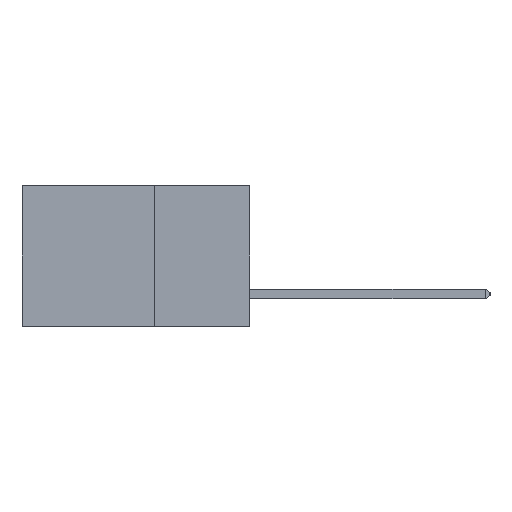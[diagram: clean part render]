
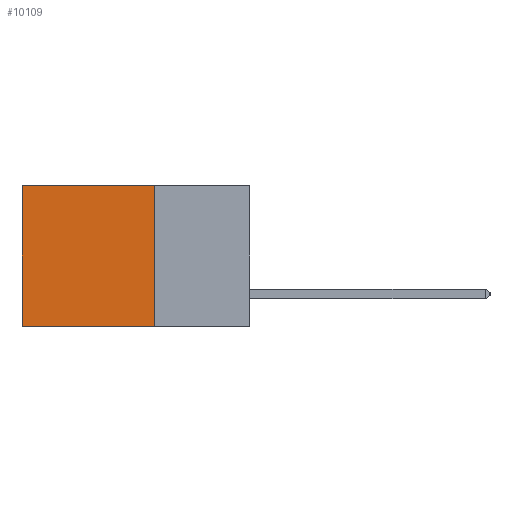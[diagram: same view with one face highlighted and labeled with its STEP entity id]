
A CAD part, left-side view. The second image highlights one B-rep face of the part: STEP entity #10109.
In plain terms, the highlighted planar face has unit normal (-1, 0, 0).
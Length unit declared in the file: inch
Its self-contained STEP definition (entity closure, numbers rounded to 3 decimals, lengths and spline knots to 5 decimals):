
#1474 = VERTEX_POINT ( 'NONE', #6374 ) ;
#2538 = CARTESIAN_POINT ( 'NONE',  ( 0.2875, 0.6, 0. ) ) ;
#4101 = ORIENTED_EDGE ( 'NONE', *, *, #33002, .T. ) ;
#6374 = CARTESIAN_POINT ( 'NONE',  ( 0.2875, 0.6, -0.37 ) ) ;
#6629 = CARTESIAN_POINT ( 'NONE',  ( 0.2875, 0.25, 0. ) ) ;
#8151 = CARTESIAN_POINT ( 'NONE',  ( 0.2875, 0.25, 0. ) ) ;
#8459 = FACE_OUTER_BOUND ( 'NONE', #9461, .T. ) ;
#9461 = EDGE_LOOP ( 'NONE', ( #17662, #22666, #15931, #4101 ) ) ;
#10109 = ADVANCED_FACE ( 'NONE', ( #8459 ), #17130, .F. ) ;
#10441 = DIRECTION ( 'NONE',  ( 1., 0., 0. ) ) ;
#10580 = DIRECTION ( 'NONE',  ( 0., 0., -1. ) ) ;
#13747 = CARTESIAN_POINT ( 'NONE',  ( 0.2875, 0.25, 0. ) ) ;
#14073 = AXIS2_PLACEMENT_3D ( 'NONE', #30080, #10441, #10580 ) ;
#14225 = VECTOR ( 'NONE', #18130, 39.37008 ) ;
#15931 = ORIENTED_EDGE ( 'NONE', *, *, #26879, .F. ) ;
#17130 = PLANE ( 'NONE',  #14073 ) ;
#17662 = ORIENTED_EDGE ( 'NONE', *, *, #18040, .T. ) ;
#18040 = EDGE_CURVE ( 'NONE', #34948, #1474, #19881, .T. ) ;
#18130 = DIRECTION ( 'NONE',  ( 0., 0., -1. ) ) ;
#19000 = CARTESIAN_POINT ( 'NONE',  ( 0.2875, 0.6, 0. ) ) ;
#19881 = LINE ( 'NONE', #19000, #23425 ) ;
#20904 = VERTEX_POINT ( 'NONE', #13747 ) ;
#21015 = VECTOR ( 'NONE', #29417, 39.37008 ) ;
#22666 = ORIENTED_EDGE ( 'NONE', *, *, #32271, .F. ) ;
#23425 = VECTOR ( 'NONE', #35064, 39.37008 ) ;
#26879 = EDGE_CURVE ( 'NONE', #20904, #33030, #35597, .T. ) ;
#28704 = LINE ( 'NONE', #6629, #21015 ) ;
#29417 = DIRECTION ( 'NONE',  ( 0., 1., 0. ) ) ;
#30080 = CARTESIAN_POINT ( 'NONE',  ( 0.2875, 0.25, 0. ) ) ;
#30247 = VECTOR ( 'NONE', #35317, 39.37008 ) ;
#32271 = EDGE_CURVE ( 'NONE', #33030, #1474, #41916, .T. ) ;
#33002 = EDGE_CURVE ( 'NONE', #20904, #34948, #28704, .T. ) ;
#33030 = VERTEX_POINT ( 'NONE', #33090 ) ;
#33090 = CARTESIAN_POINT ( 'NONE',  ( 0.2875, 0.25, -0.37 ) ) ;
#34948 = VERTEX_POINT ( 'NONE', #2538 ) ;
#35064 = DIRECTION ( 'NONE',  ( 0., 0., -1. ) ) ;
#35317 = DIRECTION ( 'NONE',  ( 0., 1., 0. ) ) ;
#35597 = LINE ( 'NONE', #8151, #14225 ) ;
#38329 = CARTESIAN_POINT ( 'NONE',  ( 0.2875, 0.25, -0.37 ) ) ;
#41916 = LINE ( 'NONE', #38329, #30247 ) ;
